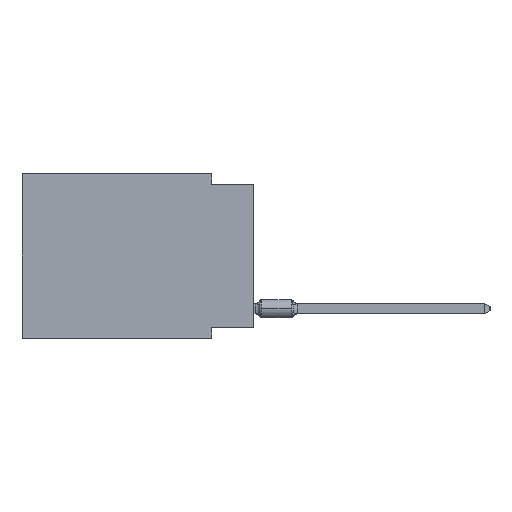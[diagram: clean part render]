
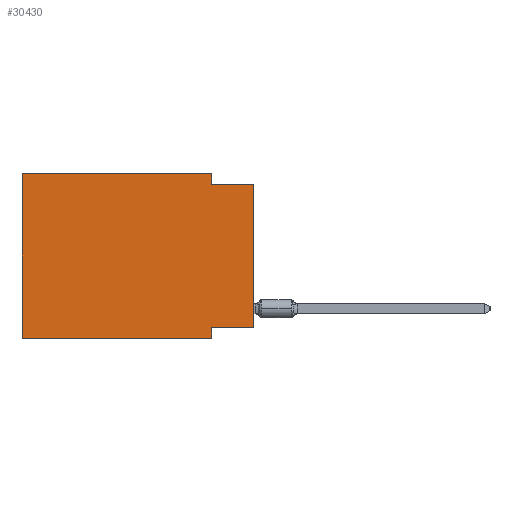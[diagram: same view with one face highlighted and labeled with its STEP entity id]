
A CAD part, left-side view. The second image highlights one B-rep face of the part: STEP entity #30430.
In plain terms, the highlighted planar face has unit normal (-1, 0, 0).
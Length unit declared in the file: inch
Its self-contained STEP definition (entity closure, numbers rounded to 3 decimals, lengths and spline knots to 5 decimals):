
#449 = ORIENTED_EDGE ( 'NONE', *, *, #13930, .F. ) ;
#535 = VECTOR ( 'NONE', #27036, 39.37008 ) ;
#3289 = ORIENTED_EDGE ( 'NONE', *, *, #10487, .F. ) ;
#6887 = LINE ( 'NONE', #55331, #13573 ) ;
#6899 = CARTESIAN_POINT ( 'NONE',  ( 0., 0.55, 0. ) ) ;
#7536 = VECTOR ( 'NONE', #53344, 39.37008 ) ;
#8378 = LINE ( 'NONE', #17695, #25386 ) ;
#10375 = AXIS2_PLACEMENT_3D ( 'NONE', #36110, #27435, #17493 ) ;
#10487 = EDGE_CURVE ( 'NONE', #61993, #30472, #51165, .T. ) ;
#12791 = CARTESIAN_POINT ( 'NONE',  ( 0., 0., -0.025 ) ) ;
#12884 = LINE ( 'NONE', #18011, #535 ) ;
#13573 = VECTOR ( 'NONE', #60487, 39.37008 ) ;
#13651 = CARTESIAN_POINT ( 'NONE',  ( 0., 0., -0.025 ) ) ;
#13930 = EDGE_CURVE ( 'NONE', #30472, #47622, #26937, .T. ) ;
#14945 = ORIENTED_EDGE ( 'NONE', *, *, #15184, .F. ) ;
#15184 = EDGE_CURVE ( 'NONE', #44217, #19866, #17616, .T. ) ;
#16317 = EDGE_CURVE ( 'NONE', #34878, #19866, #12884, .T. ) ;
#16545 = PLANE ( 'NONE',  #10375 ) ;
#16760 = CARTESIAN_POINT ( 'NONE',  ( 0., 0.55, -0.39 ) ) ;
#17493 = DIRECTION ( 'NONE',  ( 0., 0., -1. ) ) ;
#17616 = LINE ( 'NONE', #12791, #17844 ) ;
#17695 = CARTESIAN_POINT ( 'NONE',  ( 0., 0.1, -0.39 ) ) ;
#17844 = VECTOR ( 'NONE', #27563, 39.37008 ) ;
#18011 = CARTESIAN_POINT ( 'NONE',  ( 0., 0., 0. ) ) ;
#19866 = VERTEX_POINT ( 'NONE', #13651 ) ;
#20404 = CARTESIAN_POINT ( 'NONE',  ( 0., 0.1, -0.025 ) ) ;
#21546 = ORIENTED_EDGE ( 'NONE', *, *, #58388, .F. ) ;
#22106 = CARTESIAN_POINT ( 'NONE',  ( 0., 0.55, 0. ) ) ;
#24478 = CARTESIAN_POINT ( 'NONE',  ( 0., 0.1, 0. ) ) ;
#25386 = VECTOR ( 'NONE', #33081, 39.37008 ) ;
#25718 = VECTOR ( 'NONE', #45725, 39.37008 ) ;
#25869 = DIRECTION ( 'NONE',  ( 0., 1., 0. ) ) ;
#25936 = EDGE_LOOP ( 'NONE', ( #53351, #14945, #32018, #449, #3289, #34909, #35990, #21546 ) ) ;
#26937 = LINE ( 'NONE', #22106, #47487 ) ;
#27036 = DIRECTION ( 'NONE',  ( 0., 0., 1. ) ) ;
#27435 = DIRECTION ( 'NONE',  ( 1., 0., 0. ) ) ;
#27563 = DIRECTION ( 'NONE',  ( 0., -1., 0. ) ) ;
#27752 = CARTESIAN_POINT ( 'NONE',  ( 0., 0.55, 0. ) ) ;
#28285 = CARTESIAN_POINT ( 'NONE',  ( 0., 0.1, -0.39 ) ) ;
#30430 = ADVANCED_FACE ( 'NONE', ( #46069 ), #16545, .F. ) ;
#30472 = VERTEX_POINT ( 'NONE', #27752 ) ;
#32018 = ORIENTED_EDGE ( 'NONE', *, *, #61732, .F. ) ;
#33081 = DIRECTION ( 'NONE',  ( 0., 0., -1. ) ) ;
#34878 = VERTEX_POINT ( 'NONE', #41661 ) ;
#34909 = ORIENTED_EDGE ( 'NONE', *, *, #52684, .T. ) ;
#35486 = CARTESIAN_POINT ( 'NONE',  ( 0., 0., -0.365 ) ) ;
#35990 = ORIENTED_EDGE ( 'NONE', *, *, #46498, .F. ) ;
#36110 = CARTESIAN_POINT ( 'NONE',  ( 0., 0.55, 0. ) ) ;
#37110 = VERTEX_POINT ( 'NONE', #62947 ) ;
#37786 = DIRECTION ( 'NONE',  ( 0., -1., 0. ) ) ;
#41661 = CARTESIAN_POINT ( 'NONE',  ( 0., 0., -0.365 ) ) ;
#42165 = VECTOR ( 'NONE', #25869, 39.37008 ) ;
#44217 = VERTEX_POINT ( 'NONE', #20404 ) ;
#45725 = DIRECTION ( 'NONE',  ( 0., 0., 1. ) ) ;
#46069 = FACE_OUTER_BOUND ( 'NONE', #25936, .T. ) ;
#46498 = EDGE_CURVE ( 'NONE', #37110, #56083, #8378, .T. ) ;
#47487 = VECTOR ( 'NONE', #37786, 39.37008 ) ;
#47622 = VERTEX_POINT ( 'NONE', #56602 ) ;
#51165 = LINE ( 'NONE', #6899, #25718 ) ;
#52684 = EDGE_CURVE ( 'NONE', #61993, #56083, #6887, .T. ) ;
#53344 = DIRECTION ( 'NONE',  ( 0., 0., -1. ) ) ;
#53351 = ORIENTED_EDGE ( 'NONE', *, *, #16317, .T. ) ;
#55331 = CARTESIAN_POINT ( 'NONE',  ( 0., 0.55, -0.39 ) ) ;
#56083 = VERTEX_POINT ( 'NONE', #28285 ) ;
#56602 = CARTESIAN_POINT ( 'NONE',  ( 0., 0.1, 0. ) ) ;
#57228 = LINE ( 'NONE', #24478, #7536 ) ;
#58388 = EDGE_CURVE ( 'NONE', #34878, #37110, #60851, .T. ) ;
#60487 = DIRECTION ( 'NONE',  ( 0., -1., 0. ) ) ;
#60851 = LINE ( 'NONE', #35486, #42165 ) ;
#61732 = EDGE_CURVE ( 'NONE', #47622, #44217, #57228, .T. ) ;
#61993 = VERTEX_POINT ( 'NONE', #16760 ) ;
#62947 = CARTESIAN_POINT ( 'NONE',  ( 0., 0.1, -0.365 ) ) ;
